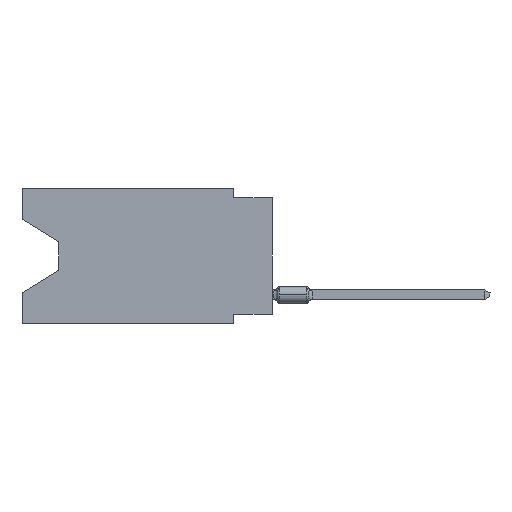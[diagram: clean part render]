
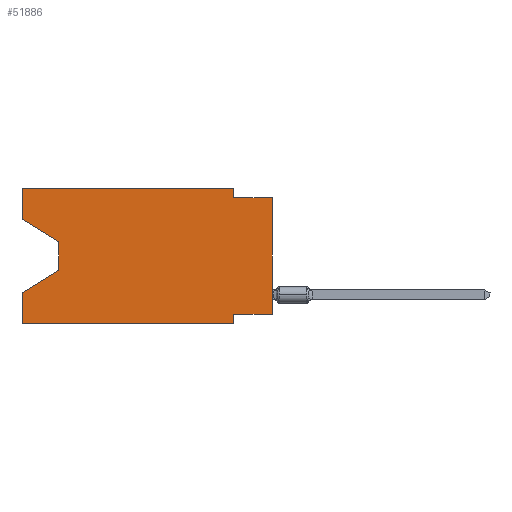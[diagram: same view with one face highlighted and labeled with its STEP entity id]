
A CAD part, left-side view. The second image highlights one B-rep face of the part: STEP entity #51886.
In plain terms, the highlighted planar face has unit normal (-1, 0, 0).
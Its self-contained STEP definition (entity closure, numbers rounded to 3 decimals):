
#383 = PLANE ( 'NONE',  #71222 ) ;
#491 = EDGE_CURVE ( 'NONE', #60037, #1267, #27006, .T. ) ;
#752 = FACE_OUTER_BOUND ( 'NONE', #62405, .T. ) ;
#810 = CARTESIAN_POINT ( 'NONE',  ( 0., 16.383, 0. ) ) ;
#1267 = VERTEX_POINT ( 'NONE', #48538 ) ;
#1720 = ORIENTED_EDGE ( 'NONE', *, *, #491, .F. ) ;
#2078 = LINE ( 'NONE', #53277, #38181 ) ;
#3947 = CARTESIAN_POINT ( 'NONE',  ( 0., 0., 0. ) ) ;
#4782 = VECTOR ( 'NONE', #71875, 1000. ) ;
#4911 = EDGE_CURVE ( 'NONE', #41678, #60037, #5330, .T. ) ;
#5330 = LINE ( 'NONE', #28123, #34085 ) ;
#5620 = DIRECTION ( 'NONE',  ( 1., 0., 0. ) ) ;
#5980 = DIRECTION ( 'NONE',  ( 0., 0., -1. ) ) ;
#7140 = EDGE_CURVE ( 'NONE', #59005, #58165, #56194, .T. ) ;
#7201 = DIRECTION ( 'NONE',  ( 0., -0.855, -0.519 ) ) ;
#9695 = VERTEX_POINT ( 'NONE', #32552 ) ;
#10262 = LINE ( 'NONE', #33044, #68072 ) ;
#12101 = VERTEX_POINT ( 'NONE', #25598 ) ;
#15252 = CARTESIAN_POINT ( 'NONE',  ( 0., 13.97, -3.505 ) ) ;
#15343 = EDGE_CURVE ( 'NONE', #58165, #54970, #2078, .T. ) ;
#16573 = DIRECTION ( 'NONE',  ( 0., 0., -1. ) ) ;
#16764 = VECTOR ( 'NONE', #7201, 1000. ) ;
#16832 = CARTESIAN_POINT ( 'NONE',  ( 0., 16.383, 0. ) ) ;
#17675 = ORIENTED_EDGE ( 'NONE', *, *, #72825, .F. ) ;
#17774 = EDGE_CURVE ( 'NONE', #9695, #48717, #22991, .T. ) ;
#18512 = DIRECTION ( 'NONE',  ( 0., 0., -1. ) ) ;
#18886 = CARTESIAN_POINT ( 'NONE',  ( 0., 2.54, 0. ) ) ;
#19436 = CARTESIAN_POINT ( 'NONE',  ( 0., 16.383, -8.89 ) ) ;
#20018 = CARTESIAN_POINT ( 'NONE',  ( 0., 16.383, -6.852 ) ) ;
#20154 = ORIENTED_EDGE ( 'NONE', *, *, #57847, .F. ) ;
#21201 = ORIENTED_EDGE ( 'NONE', *, *, #15343, .T. ) ;
#22128 = DIRECTION ( 'NONE',  ( 0., -1., 0. ) ) ;
#22543 = ORIENTED_EDGE ( 'NONE', *, *, #4911, .F. ) ;
#22991 = LINE ( 'NONE', #45424, #35861 ) ;
#23519 = CARTESIAN_POINT ( 'NONE',  ( 0., 2.54, -8.255 ) ) ;
#24031 = LINE ( 'NONE', #63665, #16764 ) ;
#25598 = CARTESIAN_POINT ( 'NONE',  ( 0., 2.54, 0. ) ) ;
#26163 = ORIENTED_EDGE ( 'NONE', *, *, #71622, .T. ) ;
#26354 = LINE ( 'NONE', #37939, #70969 ) ;
#27006 = LINE ( 'NONE', #27361, #4782 ) ;
#27361 = CARTESIAN_POINT ( 'NONE',  ( 0., 2.54, -8.89 ) ) ;
#28070 = EDGE_CURVE ( 'NONE', #52775, #54970, #10262, .T. ) ;
#28123 = CARTESIAN_POINT ( 'NONE',  ( 0., 0., -8.255 ) ) ;
#28547 = CARTESIAN_POINT ( 'NONE',  ( 0., 16.383, 0. ) ) ;
#28891 = CARTESIAN_POINT ( 'NONE',  ( 0., 13.97, -3.505 ) ) ;
#29372 = LINE ( 'NONE', #18886, #30348 ) ;
#30348 = VECTOR ( 'NONE', #18512, 1000. ) ;
#30716 = EDGE_CURVE ( 'NONE', #48717, #12101, #46379, .T. ) ;
#31716 = CARTESIAN_POINT ( 'NONE',  ( 0., 16.383, -8.89 ) ) ;
#32219 = CARTESIAN_POINT ( 'NONE',  ( 0., 2.54, -0.635 ) ) ;
#32552 = CARTESIAN_POINT ( 'NONE',  ( 0., 16.383, -2.038 ) ) ;
#32979 = CARTESIAN_POINT ( 'NONE',  ( 0., 13.97, -5.385 ) ) ;
#33044 = CARTESIAN_POINT ( 'NONE',  ( 0., 16.383, 0. ) ) ;
#34085 = VECTOR ( 'NONE', #55796, 1000. ) ;
#34783 = ORIENTED_EDGE ( 'NONE', *, *, #28070, .F. ) ;
#35861 = VECTOR ( 'NONE', #68240, 1000. ) ;
#36055 = DIRECTION ( 'NONE',  ( 0., 0.855, -0.519 ) ) ;
#36471 = VECTOR ( 'NONE', #49528, 1000. ) ;
#36955 = DIRECTION ( 'NONE',  ( 0., -1., 0. ) ) ;
#37939 = CARTESIAN_POINT ( 'NONE',  ( 0., 0., -0.635 ) ) ;
#38181 = VECTOR ( 'NONE', #36055, 1000. ) ;
#40729 = VECTOR ( 'NONE', #22128, 1000. ) ;
#41678 = VERTEX_POINT ( 'NONE', #64268 ) ;
#42562 = CARTESIAN_POINT ( 'NONE',  ( 0., 0., -0.635 ) ) ;
#43634 = ORIENTED_EDGE ( 'NONE', *, *, #17774, .F. ) ;
#45424 = CARTESIAN_POINT ( 'NONE',  ( 0., 16.383, 0. ) ) ;
#46379 = LINE ( 'NONE', #810, #40729 ) ;
#48538 = CARTESIAN_POINT ( 'NONE',  ( 0., 2.54, -8.89 ) ) ;
#48717 = VERTEX_POINT ( 'NONE', #28547 ) ;
#49148 = DIRECTION ( 'NONE',  ( 0., -1., 0. ) ) ;
#49238 = VECTOR ( 'NONE', #36955, 1000. ) ;
#49528 = DIRECTION ( 'NONE',  ( 0., 0., 1. ) ) ;
#51886 = ADVANCED_FACE ( 'NONE', ( #752 ), #383, .F. ) ;
#52775 = VERTEX_POINT ( 'NONE', #19436 ) ;
#53162 = ORIENTED_EDGE ( 'NONE', *, *, #7140, .T. ) ;
#53277 = CARTESIAN_POINT ( 'NONE',  ( 0., 13.97, -5.385 ) ) ;
#54970 = VERTEX_POINT ( 'NONE', #20018 ) ;
#55141 = LINE ( 'NONE', #3947, #36471 ) ;
#55796 = DIRECTION ( 'NONE',  ( 0., 1., 0. ) ) ;
#55861 = DIRECTION ( 'NONE',  ( 0., 0., 1. ) ) ;
#56194 = LINE ( 'NONE', #28891, #69950 ) ;
#57029 = VERTEX_POINT ( 'NONE', #32219 ) ;
#57847 = EDGE_CURVE ( 'NONE', #57029, #60221, #26354, .T. ) ;
#58165 = VERTEX_POINT ( 'NONE', #32979 ) ;
#59005 = VERTEX_POINT ( 'NONE', #15252 ) ;
#60037 = VERTEX_POINT ( 'NONE', #23519 ) ;
#60221 = VERTEX_POINT ( 'NONE', #42562 ) ;
#60619 = LINE ( 'NONE', #31716, #49238 ) ;
#60750 = EDGE_CURVE ( 'NONE', #41678, #60221, #55141, .T. ) ;
#62002 = ORIENTED_EDGE ( 'NONE', *, *, #60750, .T. ) ;
#62405 = EDGE_LOOP ( 'NONE', ( #73826, #53162, #21201, #34783, #26163, #1720, #22543, #62002, #20154, #17675, #65064, #43634 ) ) ;
#63665 = CARTESIAN_POINT ( 'NONE',  ( 0., 16.383, -2.038 ) ) ;
#64268 = CARTESIAN_POINT ( 'NONE',  ( 0., 0., -8.255 ) ) ;
#65064 = ORIENTED_EDGE ( 'NONE', *, *, #30716, .F. ) ;
#68072 = VECTOR ( 'NONE', #55861, 1000. ) ;
#68240 = DIRECTION ( 'NONE',  ( 0., 0., 1. ) ) ;
#69950 = VECTOR ( 'NONE', #16573, 1000. ) ;
#70969 = VECTOR ( 'NONE', #49148, 1000. ) ;
#71222 = AXIS2_PLACEMENT_3D ( 'NONE', #16832, #5620, #5980 ) ;
#71622 = EDGE_CURVE ( 'NONE', #52775, #1267, #60619, .T. ) ;
#71875 = DIRECTION ( 'NONE',  ( 0., 0., -1. ) ) ;
#72825 = EDGE_CURVE ( 'NONE', #12101, #57029, #29372, .T. ) ;
#73236 = EDGE_CURVE ( 'NONE', #9695, #59005, #24031, .T. ) ;
#73826 = ORIENTED_EDGE ( 'NONE', *, *, #73236, .T. ) ;
